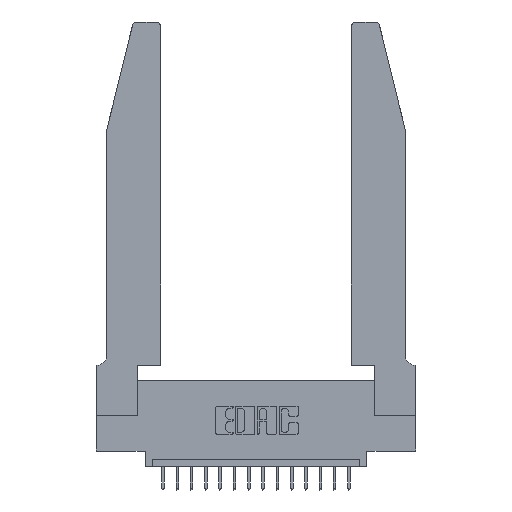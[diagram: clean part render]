
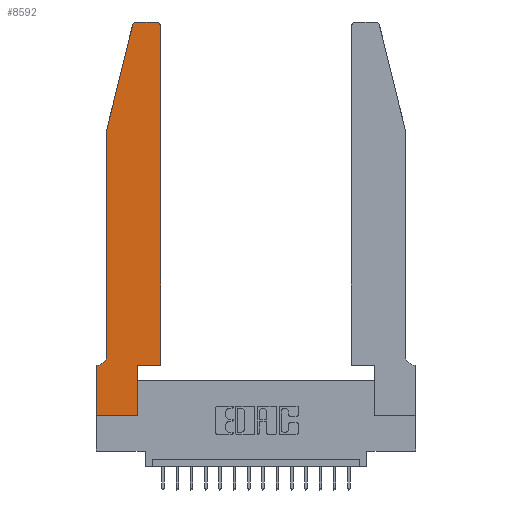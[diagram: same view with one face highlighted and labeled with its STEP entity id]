
A CAD part, top view. The second image highlights one B-rep face of the part: STEP entity #8592.
In plain terms, the highlighted planar face has unit normal (0, 0, 1).
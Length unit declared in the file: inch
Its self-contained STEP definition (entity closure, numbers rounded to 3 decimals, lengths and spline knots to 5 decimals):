
#484 = CARTESIAN_POINT ( 'NONE',  ( 0.0755, 2., 0.37 ) ) ;
#847 = VERTEX_POINT ( 'NONE', #6657 ) ;
#949 = ORIENTED_EDGE ( 'NONE', *, *, #17345, .T. ) ;
#1060 = EDGE_CURVE ( 'NONE', #8672, #9027, #9600, .T. ) ;
#1163 = AXIS2_PLACEMENT_3D ( 'NONE', #16339, #7435, #3155 ) ;
#1307 = DIRECTION ( 'NONE',  ( 0., 0., -1. ) ) ;
#1365 = VERTEX_POINT ( 'NONE', #18034 ) ;
#1413 = DIRECTION ( 'NONE',  ( -0.239, -0.971, 0. ) ) ;
#1500 = CARTESIAN_POINT ( 'NONE',  ( 0., 0., 0.37 ) ) ;
#1544 = LINE ( 'NONE', #484, #14553 ) ;
#1802 = ORIENTED_EDGE ( 'NONE', *, *, #1060, .T. ) ;
#2447 = CIRCLE ( 'NONE', #11984, 0.07 ) ;
#2508 = VERTEX_POINT ( 'NONE', #7979 ) ;
#2795 = DIRECTION ( 'NONE',  ( -1., 0., 0. ) ) ;
#3155 = DIRECTION ( 'NONE',  ( 1., 0., 0. ) ) ;
#3257 = ORIENTED_EDGE ( 'NONE', *, *, #9847, .T. ) ;
#3574 = ORIENTED_EDGE ( 'NONE', *, *, #15023, .T. ) ;
#4060 = VECTOR ( 'NONE', #1413, 39.37008 ) ;
#4064 = VERTEX_POINT ( 'NONE', #7977 ) ;
#4324 = CARTESIAN_POINT ( 'NONE',  ( 0.0055, 0.35, 0.37 ) ) ;
#4363 = AXIS2_PLACEMENT_3D ( 'NONE', #14449, #10008, #7087 ) ;
#5402 = CARTESIAN_POINT ( 'NONE',  ( 0.0755, 0.42, 0.37 ) ) ;
#5641 = CARTESIAN_POINT ( 'NONE',  ( 0.0055, 0.42, 0.37 ) ) ;
#5762 = DIRECTION ( 'NONE',  ( 1., 0., 0. ) ) ;
#5789 = EDGE_CURVE ( 'NONE', #18798, #847, #10819, .T. ) ;
#6489 = DIRECTION ( 'NONE',  ( 1., 0., 0. ) ) ;
#6573 = VECTOR ( 'NONE', #11096, 39.37008 ) ;
#6657 = CARTESIAN_POINT ( 'NONE',  ( 0.4505, 0.35, 0.37 ) ) ;
#7087 = DIRECTION ( 'NONE',  ( 1., 0., 0. ) ) ;
#7108 = CARTESIAN_POINT ( 'NONE',  ( 0.0755, 2., 0.37 ) ) ;
#7112 = VERTEX_POINT ( 'NONE', #18488 ) ;
#7226 = EDGE_CURVE ( 'NONE', #16684, #2508, #14453, .T. ) ;
#7317 = LINE ( 'NONE', #10483, #17107 ) ;
#7435 = DIRECTION ( 'NONE',  ( 0., 0., 1. ) ) ;
#7550 = DIRECTION ( 'NONE',  ( 1., 0., 0. ) ) ;
#7809 = DIRECTION ( 'NONE',  ( 0., 0., 1. ) ) ;
#7833 = LINE ( 'NONE', #12457, #16196 ) ;
#7977 = CARTESIAN_POINT ( 'NONE',  ( 0.25487, 2.72718, 0.37 ) ) ;
#7979 = CARTESIAN_POINT ( 'NONE',  ( 0.4205, 2.75, 0.37 ) ) ;
#8146 = DIRECTION ( 'NONE',  ( 0., -1., 0. ) ) ;
#8592 = ADVANCED_FACE ( 'NONE', ( #10657 ), #11835, .T. ) ;
#8672 = VERTEX_POINT ( 'NONE', #9170 ) ;
#9027 = VERTEX_POINT ( 'NONE', #17374 ) ;
#9132 = VECTOR ( 'NONE', #5762, 39.37008 ) ;
#9170 = CARTESIAN_POINT ( 'NONE',  ( 0., 0., 0.37 ) ) ;
#9201 = AXIS2_PLACEMENT_3D ( 'NONE', #13722, #7809, #7550 ) ;
#9296 = CARTESIAN_POINT ( 'NONE',  ( 0.2865, 0.35, 0.37 ) ) ;
#9364 = LINE ( 'NONE', #18929, #6573 ) ;
#9391 = LINE ( 'NONE', #10278, #14294 ) ;
#9600 = LINE ( 'NONE', #1500, #9132 ) ;
#9847 = EDGE_CURVE ( 'NONE', #9027, #18798, #7833, .T. ) ;
#10008 = DIRECTION ( 'NONE',  ( 0., 0., 1. ) ) ;
#10045 = CARTESIAN_POINT ( 'NONE',  ( 0.4505, 2.72, 0.37 ) ) ;
#10247 = ORIENTED_EDGE ( 'NONE', *, *, #10647, .T. ) ;
#10278 = CARTESIAN_POINT ( 'NONE',  ( 0.4505, 0.35, 0.37 ) ) ;
#10432 = ORIENTED_EDGE ( 'NONE', *, *, #12667, .T. ) ;
#10483 = CARTESIAN_POINT ( 'NONE',  ( 0.2605, 2.75, 0.37 ) ) ;
#10647 = EDGE_CURVE ( 'NONE', #1365, #12099, #1544, .T. ) ;
#10657 = FACE_OUTER_BOUND ( 'NONE', #11721, .T. ) ;
#10819 = LINE ( 'NONE', #13927, #17825 ) ;
#10968 = EDGE_CURVE ( 'NONE', #12099, #14594, #2447, .T. ) ;
#10983 = CARTESIAN_POINT ( 'NONE',  ( 0., 0.35, 0.37 ) ) ;
#11096 = DIRECTION ( 'NONE',  ( -1., 0., 0. ) ) ;
#11133 = DIRECTION ( 'NONE',  ( 0., -1., 0. ) ) ;
#11631 = EDGE_CURVE ( 'NONE', #4064, #1365, #11937, .T. ) ;
#11721 = EDGE_LOOP ( 'NONE', ( #15274, #17057, #13426, #10247, #13057, #10432, #3574, #1802, #3257, #17155, #949, #12453 ) ) ;
#11835 = PLANE ( 'NONE',  #1163 ) ;
#11937 = LINE ( 'NONE', #7108, #4060 ) ;
#11984 = AXIS2_PLACEMENT_3D ( 'NONE', #5641, #1307, #2795 ) ;
#12048 = DIRECTION ( 'NONE',  ( -1., 0., 0. ) ) ;
#12099 = VERTEX_POINT ( 'NONE', #5402 ) ;
#12254 = DIRECTION ( 'NONE',  ( 0., 1., 0. ) ) ;
#12453 = ORIENTED_EDGE ( 'NONE', *, *, #7226, .T. ) ;
#12457 = CARTESIAN_POINT ( 'NONE',  ( 0.2865, 0.35, 0.37 ) ) ;
#12667 = EDGE_CURVE ( 'NONE', #14594, #13780, #9364, .T. ) ;
#13057 = ORIENTED_EDGE ( 'NONE', *, *, #10968, .T. ) ;
#13426 = ORIENTED_EDGE ( 'NONE', *, *, #11631, .T. ) ;
#13722 = CARTESIAN_POINT ( 'NONE',  ( 0.284, 2.72, 0.37 ) ) ;
#13780 = VERTEX_POINT ( 'NONE', #10983 ) ;
#13927 = CARTESIAN_POINT ( 'NONE',  ( 0.4505, 0.35, 0.37 ) ) ;
#13945 = CARTESIAN_POINT ( 'NONE',  ( 0., 0., 0.37 ) ) ;
#14294 = VECTOR ( 'NONE', #19291, 39.37008 ) ;
#14449 = CARTESIAN_POINT ( 'NONE',  ( 0.4205, 2.72, 0.37 ) ) ;
#14453 = CIRCLE ( 'NONE', #4363, 0.03 ) ;
#14553 = VECTOR ( 'NONE', #8146, 39.37008 ) ;
#14594 = VERTEX_POINT ( 'NONE', #4324 ) ;
#15023 = EDGE_CURVE ( 'NONE', #13780, #8672, #15363, .T. ) ;
#15274 = ORIENTED_EDGE ( 'NONE', *, *, #16915, .T. ) ;
#15363 = LINE ( 'NONE', #13945, #16951 ) ;
#15846 = EDGE_CURVE ( 'NONE', #7112, #4064, #16434, .T. ) ;
#16196 = VECTOR ( 'NONE', #12254, 39.37008 ) ;
#16339 = CARTESIAN_POINT ( 'NONE',  ( 0., 0.35, 0.37 ) ) ;
#16434 = CIRCLE ( 'NONE', #9201, 0.03 ) ;
#16684 = VERTEX_POINT ( 'NONE', #10045 ) ;
#16915 = EDGE_CURVE ( 'NONE', #2508, #7112, #7317, .T. ) ;
#16951 = VECTOR ( 'NONE', #11133, 39.37008 ) ;
#17057 = ORIENTED_EDGE ( 'NONE', *, *, #15846, .T. ) ;
#17107 = VECTOR ( 'NONE', #12048, 39.37008 ) ;
#17155 = ORIENTED_EDGE ( 'NONE', *, *, #5789, .T. ) ;
#17345 = EDGE_CURVE ( 'NONE', #847, #16684, #9391, .T. ) ;
#17374 = CARTESIAN_POINT ( 'NONE',  ( 0.2865, 0., 0.37 ) ) ;
#17825 = VECTOR ( 'NONE', #6489, 39.37008 ) ;
#18034 = CARTESIAN_POINT ( 'NONE',  ( 0.0755, 2., 0.37 ) ) ;
#18488 = CARTESIAN_POINT ( 'NONE',  ( 0.284, 2.75, 0.37 ) ) ;
#18798 = VERTEX_POINT ( 'NONE', #9296 ) ;
#18929 = CARTESIAN_POINT ( 'NONE',  ( 0.0755, 0.35, 0.37 ) ) ;
#19291 = DIRECTION ( 'NONE',  ( 0., 1., 0. ) ) ;
